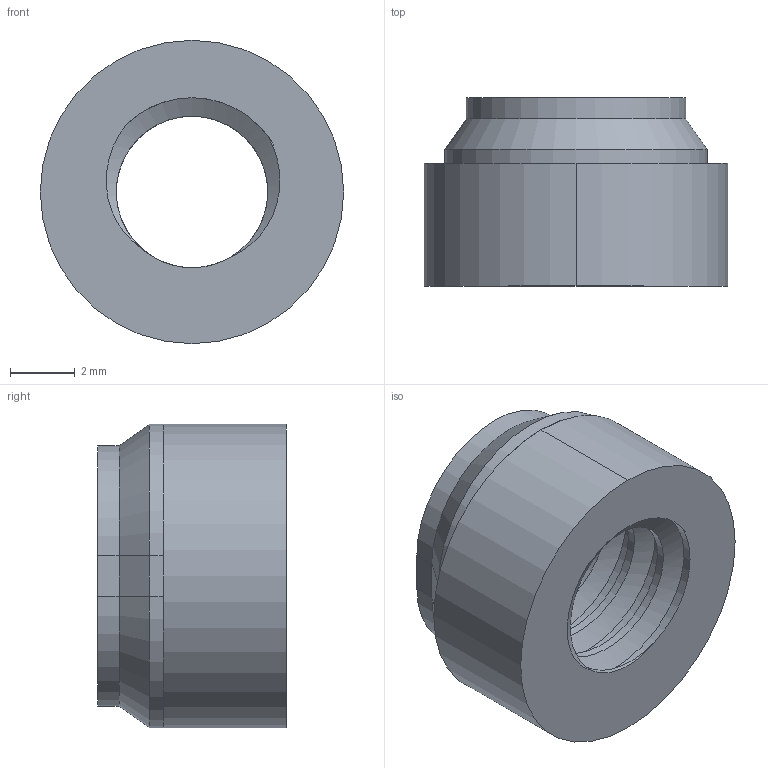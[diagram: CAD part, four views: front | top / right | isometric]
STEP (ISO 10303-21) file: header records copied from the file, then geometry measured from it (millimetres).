
FILE_DESCRIPTION (( 'STEP AP203' ), '1' );
FILE_NAME ('AF-WF-VF-PRT-003-STEP.STEP', '2020-07-22T01:00:17', ( '' ), ( '' ), 'SwSTEP 2.0', 'SolidWorks 2018', '' );
FILE_SCHEMA (( 'CONFIG_CONTROL_DESIGN' ));
Length unit declared in the file: inch
Products named in the file (1): AF-WF-VF-PRT-003-STEP
Bounding box: 9.4 x 5.84 x 9.4 mm (x, y, z)
Volume: 239 mm3; surface area: 387.8 mm2
Topology: 1 solids, 1 shells, 36 faces, 85 edges, 51 vertices
Faces by surface type: cylinder 19, plane 11, cone 3, bspline 3
Entity records: 1823 total; most frequent: CARTESIAN_POINT 979, ORIENTED_EDGE 170, DIRECTION 151, EDGE_CURVE 85, AXIS2_PLACEMENT_3D 56, VERTEX_POINT 51, LINE 39, VECTOR 39
